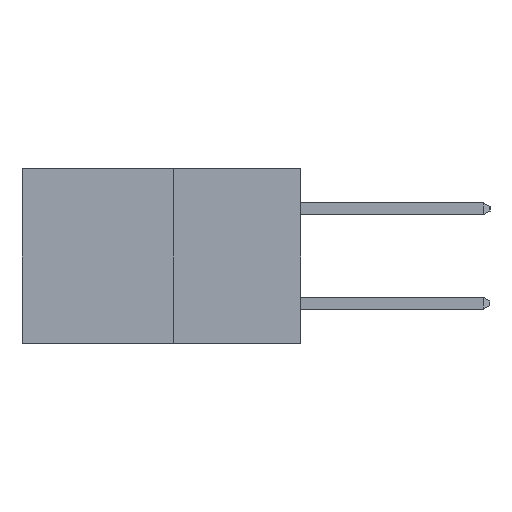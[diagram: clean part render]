
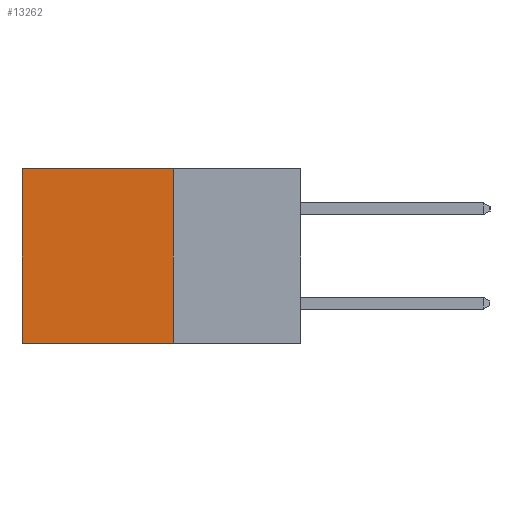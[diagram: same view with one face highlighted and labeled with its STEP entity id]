
A CAD part, left-side view. The second image highlights one B-rep face of the part: STEP entity #13262.
In plain terms, the highlighted planar face has unit normal (-1, 0, 0).
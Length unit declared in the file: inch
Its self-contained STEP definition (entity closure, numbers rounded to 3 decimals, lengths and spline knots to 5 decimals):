
#1030 = VERTEX_POINT ( 'NONE', #3782 ) ;
#1100 = VECTOR ( 'NONE', #7702, 39.37008 ) ;
#1413 = EDGE_CURVE ( 'NONE', #10024, #19910, #10824, .T. ) ;
#1672 = LINE ( 'NONE', #16723, #1100 ) ;
#1724 = VECTOR ( 'NONE', #11122, 39.37008 ) ;
#3782 = CARTESIAN_POINT ( 'NONE',  ( 0.277, 0.59, 0. ) ) ;
#5101 = CARTESIAN_POINT ( 'NONE',  ( 0.277, 0.27, -0.37 ) ) ;
#5524 = ORIENTED_EDGE ( 'NONE', *, *, #21315, .F. ) ;
#5697 = DIRECTION ( 'NONE',  ( 0., 0., -1. ) ) ;
#7702 = DIRECTION ( 'NONE',  ( 0., 1., 0. ) ) ;
#9296 = CARTESIAN_POINT ( 'NONE',  ( 0.277, 0.59, -0.37 ) ) ;
#9502 = DIRECTION ( 'NONE',  ( 0., 0., -1. ) ) ;
#10024 = VERTEX_POINT ( 'NONE', #13424 ) ;
#10824 = LINE ( 'NONE', #5101, #15659 ) ;
#11122 = DIRECTION ( 'NONE',  ( 0., 0., -1. ) ) ;
#11551 = LINE ( 'NONE', #20213, #22333 ) ;
#11903 = EDGE_CURVE ( 'NONE', #1030, #19910, #20470, .T. ) ;
#11973 = AXIS2_PLACEMENT_3D ( 'NONE', #18542, #20373, #9502 ) ;
#12059 = CARTESIAN_POINT ( 'NONE',  ( 0.277, 0.27, 0. ) ) ;
#12278 = VERTEX_POINT ( 'NONE', #12059 ) ;
#13262 = ADVANCED_FACE ( 'NONE', ( #15560 ), #16695, .F. ) ;
#13424 = CARTESIAN_POINT ( 'NONE',  ( 0.277, 0.27, -0.37 ) ) ;
#13607 = ORIENTED_EDGE ( 'NONE', *, *, #11903, .T. ) ;
#15560 = FACE_OUTER_BOUND ( 'NONE', #16201, .T. ) ;
#15659 = VECTOR ( 'NONE', #19941, 39.37008 ) ;
#16201 = EDGE_LOOP ( 'NONE', ( #13607, #19208, #5524, #23315 ) ) ;
#16695 = PLANE ( 'NONE',  #11973 ) ;
#16723 = CARTESIAN_POINT ( 'NONE',  ( 0.277, 0.27, 0. ) ) ;
#18542 = CARTESIAN_POINT ( 'NONE',  ( 0.277, 0.27, -0.37 ) ) ;
#19208 = ORIENTED_EDGE ( 'NONE', *, *, #1413, .F. ) ;
#19910 = VERTEX_POINT ( 'NONE', #20971 ) ;
#19941 = DIRECTION ( 'NONE',  ( 0., 1., 0. ) ) ;
#20213 = CARTESIAN_POINT ( 'NONE',  ( 0.277, 0.27, -0.37 ) ) ;
#20373 = DIRECTION ( 'NONE',  ( 1., 0., 0. ) ) ;
#20470 = LINE ( 'NONE', #9296, #1724 ) ;
#20686 = EDGE_CURVE ( 'NONE', #12278, #1030, #1672, .T. ) ;
#20971 = CARTESIAN_POINT ( 'NONE',  ( 0.277, 0.59, -0.37 ) ) ;
#21315 = EDGE_CURVE ( 'NONE', #12278, #10024, #11551, .T. ) ;
#22333 = VECTOR ( 'NONE', #5697, 39.37008 ) ;
#23315 = ORIENTED_EDGE ( 'NONE', *, *, #20686, .T. ) ;
